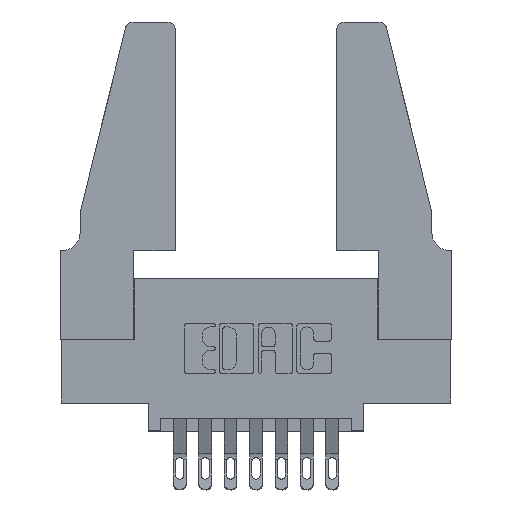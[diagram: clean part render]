
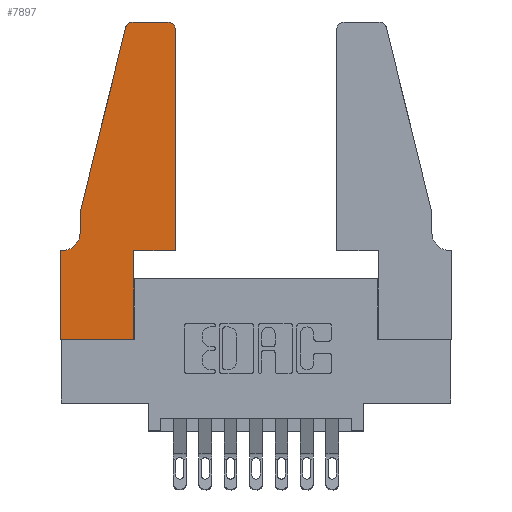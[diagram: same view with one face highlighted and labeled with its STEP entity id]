
A CAD part, top view. The second image highlights one B-rep face of the part: STEP entity #7897.
In plain terms, the highlighted planar face has unit normal (0, 0, 1).
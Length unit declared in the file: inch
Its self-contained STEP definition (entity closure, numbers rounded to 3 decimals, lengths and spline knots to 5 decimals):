
#57 = CARTESIAN_POINT ( 'NONE',  ( 0.284, 1.25, 0.37 ) ) ;
#162 = VECTOR ( 'NONE', #3880, 39.37008 ) ;
#217 = EDGE_CURVE ( 'NONE', #3738, #4131, #8125, .T. ) ;
#363 = VECTOR ( 'NONE', #3368, 39.37008 ) ;
#405 = EDGE_CURVE ( 'NONE', #1453, #1946, #2883, .T. ) ;
#538 = DIRECTION ( 'NONE',  ( 1., 0., 0. ) ) ;
#710 = VERTEX_POINT ( 'NONE', #1151 ) ;
#883 = DIRECTION ( 'NONE',  ( 1., 0., 0. ) ) ;
#889 = CARTESIAN_POINT ( 'NONE',  ( 0., 0., 0.37 ) ) ;
#904 = ORIENTED_EDGE ( 'NONE', *, *, #217, .T. ) ;
#910 = EDGE_CURVE ( 'NONE', #4131, #2414, #1008, .T. ) ;
#1008 = LINE ( 'NONE', #4804, #7645 ) ;
#1075 = CARTESIAN_POINT ( 'NONE',  ( 0.2605, 1.25, 0.37 ) ) ;
#1096 = EDGE_CURVE ( 'NONE', #8873, #12281, #11884, .T. ) ;
#1151 = CARTESIAN_POINT ( 'NONE',  ( 0., 0.35, 0.37 ) ) ;
#1298 = CARTESIAN_POINT ( 'NONE',  ( 0.2865, 0.35, 0.37 ) ) ;
#1309 = ORIENTED_EDGE ( 'NONE', *, *, #910, .T. ) ;
#1453 = VERTEX_POINT ( 'NONE', #12586 ) ;
#1604 = DIRECTION ( 'NONE',  ( -1., 0., 0. ) ) ;
#1756 = VECTOR ( 'NONE', #4966, 39.37008 ) ;
#1864 = CARTESIAN_POINT ( 'NONE',  ( 0.4505, 1.22, 0.37 ) ) ;
#1876 = CARTESIAN_POINT ( 'NONE',  ( 0.4205, 1.22, 0.37 ) ) ;
#1934 = EDGE_CURVE ( 'NONE', #2414, #2451, #9961, .T. ) ;
#1946 = VERTEX_POINT ( 'NONE', #8982 ) ;
#2288 = VERTEX_POINT ( 'NONE', #4417 ) ;
#2414 = VERTEX_POINT ( 'NONE', #5697 ) ;
#2451 = VERTEX_POINT ( 'NONE', #1864 ) ;
#2769 = VECTOR ( 'NONE', #5027, 39.37008 ) ;
#2883 = CIRCLE ( 'NONE', #5559, 0.07 ) ;
#2933 = EDGE_CURVE ( 'NONE', #710, #2288, #8069, .T. ) ;
#3214 = VECTOR ( 'NONE', #4783, 39.37008 ) ;
#3368 = DIRECTION ( 'NONE',  ( 0., 1., 0. ) ) ;
#3438 = VECTOR ( 'NONE', #5924, 39.37008 ) ;
#3540 = CARTESIAN_POINT ( 'NONE',  ( 0.0055, 0.42, 0.37 ) ) ;
#3592 = CARTESIAN_POINT ( 'NONE',  ( 0.0755, 0.5, 0.37 ) ) ;
#3738 = VERTEX_POINT ( 'NONE', #4717 ) ;
#3795 = CARTESIAN_POINT ( 'NONE',  ( 0.0755, 0.35, 0.37 ) ) ;
#3880 = DIRECTION ( 'NONE',  ( 0., -1., 0. ) ) ;
#3894 = ORIENTED_EDGE ( 'NONE', *, *, #1096, .T. ) ;
#3900 = DIRECTION ( 'NONE',  ( 0., 0., 1. ) ) ;
#3956 = CARTESIAN_POINT ( 'NONE',  ( 0., 0., 0.37 ) ) ;
#3967 = AXIS2_PLACEMENT_3D ( 'NONE', #1876, #3900, #11774 ) ;
#3977 = CARTESIAN_POINT ( 'NONE',  ( 0.4505, 0.35, 0.37 ) ) ;
#4091 = CARTESIAN_POINT ( 'NONE',  ( 0.0755, 0.5, 0.37 ) ) ;
#4131 = VERTEX_POINT ( 'NONE', #10406 ) ;
#4417 = CARTESIAN_POINT ( 'NONE',  ( 0., 0., 0.37 ) ) ;
#4561 = DIRECTION ( 'NONE',  ( 0., -1., 0. ) ) ;
#4700 = FACE_OUTER_BOUND ( 'NONE', #12716, .T. ) ;
#4717 = CARTESIAN_POINT ( 'NONE',  ( 0.2865, 0., 0.37 ) ) ;
#4783 = DIRECTION ( 'NONE',  ( -1., 0., 0. ) ) ;
#4804 = CARTESIAN_POINT ( 'NONE',  ( 0.4505, 0.35, 0.37 ) ) ;
#4889 = EDGE_CURVE ( 'NONE', #2451, #7983, #10063, .T. ) ;
#4931 = PLANE ( 'NONE',  #8185 ) ;
#4966 = DIRECTION ( 'NONE',  ( 0., 1., 0. ) ) ;
#5027 = DIRECTION ( 'NONE',  ( 1., 0., 0. ) ) ;
#5175 = DIRECTION ( 'NONE',  ( 0., 0., 1. ) ) ;
#5469 = EDGE_CURVE ( 'NONE', #1946, #710, #6793, .T. ) ;
#5559 = AXIS2_PLACEMENT_3D ( 'NONE', #3540, #6490, #1604 ) ;
#5697 = CARTESIAN_POINT ( 'NONE',  ( 0.4505, 0.35, 0.37 ) ) ;
#5750 = VERTEX_POINT ( 'NONE', #57 ) ;
#5768 = DIRECTION ( 'NONE',  ( 0., 0., 1. ) ) ;
#5869 = ORIENTED_EDGE ( 'NONE', *, *, #4889, .T. ) ;
#5924 = DIRECTION ( 'NONE',  ( -1., 0., 0. ) ) ;
#6325 = ORIENTED_EDGE ( 'NONE', *, *, #1934, .T. ) ;
#6490 = DIRECTION ( 'NONE',  ( 0., 0., -1. ) ) ;
#6721 = LINE ( 'NONE', #1075, #3438 ) ;
#6793 = LINE ( 'NONE', #3795, #3214 ) ;
#6803 = CARTESIAN_POINT ( 'NONE',  ( 0., 0.35, 0.37 ) ) ;
#6816 = AXIS2_PLACEMENT_3D ( 'NONE', #8357, #5175, #538 ) ;
#7013 = VECTOR ( 'NONE', #4561, 39.37008 ) ;
#7044 = ORIENTED_EDGE ( 'NONE', *, *, #405, .T. ) ;
#7645 = VECTOR ( 'NONE', #883, 39.37008 ) ;
#7795 = DIRECTION ( 'NONE',  ( 1., 0., 0. ) ) ;
#7897 = ADVANCED_FACE ( 'NONE', ( #4700 ), #4931, .T. ) ;
#7945 = LINE ( 'NONE', #9563, #7013 ) ;
#7983 = VERTEX_POINT ( 'NONE', #8469 ) ;
#8004 = ORIENTED_EDGE ( 'NONE', *, *, #8378, .T. ) ;
#8069 = LINE ( 'NONE', #889, #162 ) ;
#8125 = LINE ( 'NONE', #1298, #363 ) ;
#8185 = AXIS2_PLACEMENT_3D ( 'NONE', #6803, #5768, #7795 ) ;
#8328 = ORIENTED_EDGE ( 'NONE', *, *, #5469, .T. ) ;
#8357 = CARTESIAN_POINT ( 'NONE',  ( 0.284, 1.22, 0.37 ) ) ;
#8378 = EDGE_CURVE ( 'NONE', #12281, #1453, #7945, .T. ) ;
#8469 = CARTESIAN_POINT ( 'NONE',  ( 0.4205, 1.25, 0.37 ) ) ;
#8519 = LINE ( 'NONE', #3956, #2769 ) ;
#8873 = VERTEX_POINT ( 'NONE', #9973 ) ;
#8922 = VECTOR ( 'NONE', #11095, 39.37008 ) ;
#8935 = EDGE_CURVE ( 'NONE', #2288, #3738, #8519, .T. ) ;
#8982 = CARTESIAN_POINT ( 'NONE',  ( 0.0055, 0.35, 0.37 ) ) ;
#9028 = ORIENTED_EDGE ( 'NONE', *, *, #9543, .T. ) ;
#9194 = ORIENTED_EDGE ( 'NONE', *, *, #8935, .T. ) ;
#9421 = ORIENTED_EDGE ( 'NONE', *, *, #2933, .T. ) ;
#9543 = EDGE_CURVE ( 'NONE', #7983, #5750, #6721, .T. ) ;
#9563 = CARTESIAN_POINT ( 'NONE',  ( 0.0755, 0.5, 0.37 ) ) ;
#9961 = LINE ( 'NONE', #3977, #1756 ) ;
#9973 = CARTESIAN_POINT ( 'NONE',  ( 0.25487, 1.22718, 0.37 ) ) ;
#10063 = CIRCLE ( 'NONE', #3967, 0.03 ) ;
#10406 = CARTESIAN_POINT ( 'NONE',  ( 0.2865, 0.35, 0.37 ) ) ;
#11095 = DIRECTION ( 'NONE',  ( -0.239, -0.971, 0. ) ) ;
#11388 = EDGE_CURVE ( 'NONE', #5750, #8873, #12261, .T. ) ;
#11774 = DIRECTION ( 'NONE',  ( 1., 0., 0. ) ) ;
#11884 = LINE ( 'NONE', #4091, #8922 ) ;
#11976 = ORIENTED_EDGE ( 'NONE', *, *, #11388, .T. ) ;
#12261 = CIRCLE ( 'NONE', #6816, 0.03 ) ;
#12281 = VERTEX_POINT ( 'NONE', #3592 ) ;
#12586 = CARTESIAN_POINT ( 'NONE',  ( 0.0755, 0.42, 0.37 ) ) ;
#12716 = EDGE_LOOP ( 'NONE', ( #9028, #11976, #3894, #8004, #7044, #8328, #9421, #9194, #904, #1309, #6325, #5869 ) ) ;
